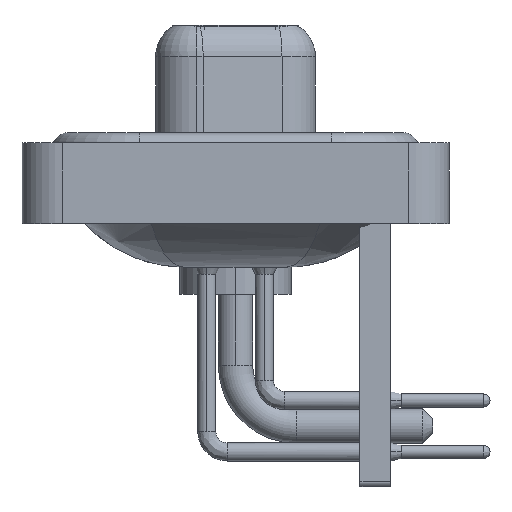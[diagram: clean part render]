
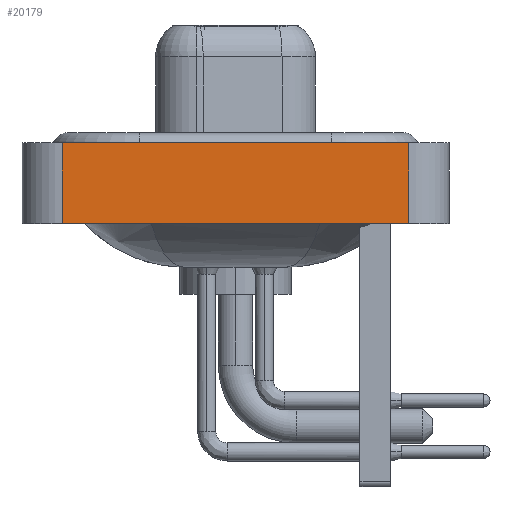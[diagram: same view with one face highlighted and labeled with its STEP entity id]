
A CAD part, left-side view. The second image highlights one B-rep face of the part: STEP entity #20179.
In plain terms, the highlighted planar face has unit normal (-1, 0, 0).
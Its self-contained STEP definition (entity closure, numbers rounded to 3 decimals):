
#70 = CARTESIAN_POINT ( 'NONE',  ( -7.3, 8.55, -3.6 ) ) ;
#1697 = EDGE_LOOP ( 'NONE', ( #15914, #4442, #7677, #2634 ) ) ;
#1921 = LINE ( 'NONE', #70, #8066 ) ;
#1933 = VERTEX_POINT ( 'NONE', #10983 ) ;
#1938 = CARTESIAN_POINT ( 'NONE',  ( -7.3, -8.55, 0.4 ) ) ;
#2445 = DIRECTION ( 'NONE',  ( 0., 0., 1. ) ) ;
#2560 = CARTESIAN_POINT ( 'NONE',  ( -7.3, -8.55, -3.6 ) ) ;
#2634 = ORIENTED_EDGE ( 'NONE', *, *, #15322, .T. ) ;
#3590 = DIRECTION ( 'NONE',  ( 0., -1., 0. ) ) ;
#3773 = CARTESIAN_POINT ( 'NONE',  ( -7.3, 8.55, 0.4 ) ) ;
#4442 = ORIENTED_EDGE ( 'NONE', *, *, #19496, .F. ) ;
#4486 = CARTESIAN_POINT ( 'NONE',  ( -7.3, -8.55, -3.6 ) ) ;
#4967 = DIRECTION ( 'NONE',  ( 0., 0., 1. ) ) ;
#6376 = LINE ( 'NONE', #4486, #17789 ) ;
#6380 = CARTESIAN_POINT ( 'NONE',  ( -7.3, -8.55, 0.4 ) ) ;
#6889 = LINE ( 'NONE', #1938, #22959 ) ;
#7510 = VERTEX_POINT ( 'NONE', #3773 ) ;
#7677 = ORIENTED_EDGE ( 'NONE', *, *, #12304, .F. ) ;
#8066 = VECTOR ( 'NONE', #10522, 1000. ) ;
#8409 = LINE ( 'NONE', #22581, #14035 ) ;
#10522 = DIRECTION ( 'NONE',  ( 0., 0., 1. ) ) ;
#10983 = CARTESIAN_POINT ( 'NONE',  ( -7.3, 8.55, -3.6 ) ) ;
#11504 = DIRECTION ( 'NONE',  ( -1., 0., 0. ) ) ;
#11927 = DIRECTION ( 'NONE',  ( 0., -1., 0. ) ) ;
#12304 = EDGE_CURVE ( 'NONE', #1933, #7510, #1921, .T. ) ;
#12633 = EDGE_CURVE ( 'NONE', #16023, #14069, #6376, .T. ) ;
#13363 = FACE_OUTER_BOUND ( 'NONE', #1697, .T. ) ;
#14035 = VECTOR ( 'NONE', #11927, 1000. ) ;
#14069 = VERTEX_POINT ( 'NONE', #6380 ) ;
#15322 = EDGE_CURVE ( 'NONE', #1933, #16023, #8409, .T. ) ;
#15914 = ORIENTED_EDGE ( 'NONE', *, *, #12633, .T. ) ;
#16023 = VERTEX_POINT ( 'NONE', #18827 ) ;
#17789 = VECTOR ( 'NONE', #4967, 1000. ) ;
#18827 = CARTESIAN_POINT ( 'NONE',  ( -7.3, -8.55, -3.6 ) ) ;
#18853 = PLANE ( 'NONE',  #19887 ) ;
#19496 = EDGE_CURVE ( 'NONE', #7510, #14069, #6889, .T. ) ;
#19887 = AXIS2_PLACEMENT_3D ( 'NONE', #2560, #11504, #2445 ) ;
#20179 = ADVANCED_FACE ( 'NONE', ( #13363 ), #18853, .T. ) ;
#22581 = CARTESIAN_POINT ( 'NONE',  ( -7.3, -8.55, -3.6 ) ) ;
#22959 = VECTOR ( 'NONE', #3590, 1000. ) ;
